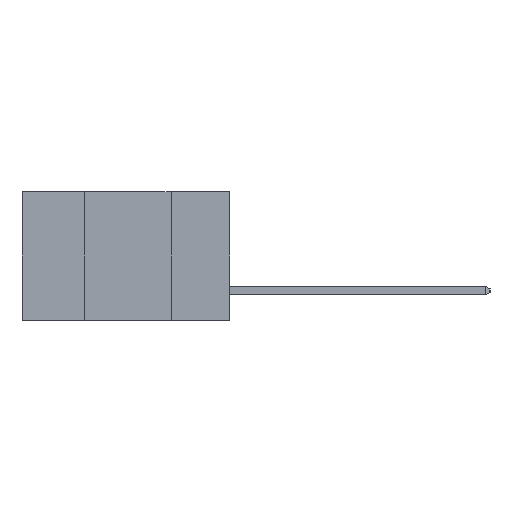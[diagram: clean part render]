
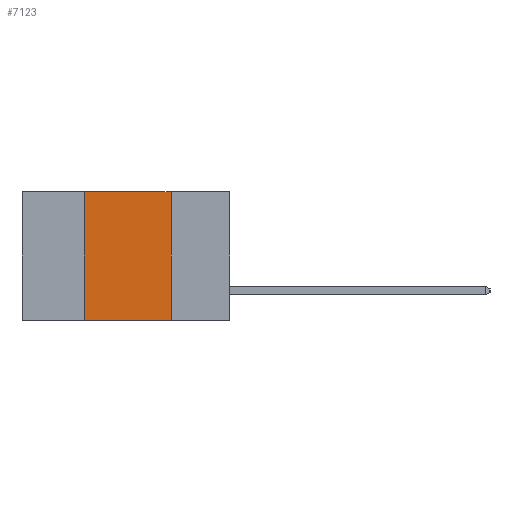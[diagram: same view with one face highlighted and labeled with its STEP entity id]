
A CAD part, left-side view. The second image highlights one B-rep face of the part: STEP entity #7123.
In plain terms, the highlighted planar face has unit normal (-1, 0, 0).
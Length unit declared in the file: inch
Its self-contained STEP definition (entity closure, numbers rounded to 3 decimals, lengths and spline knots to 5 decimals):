
#439 = ORIENTED_EDGE ( 'NONE', *, *, #2695, .F. ) ;
#980 = CARTESIAN_POINT ( 'NONE',  ( 0., 0.6, -0.37 ) ) ;
#1208 = CARTESIAN_POINT ( 'NONE',  ( 0., 0.17, -0.37 ) ) ;
#1499 = CARTESIAN_POINT ( 'NONE',  ( 0., 0.17, 0. ) ) ;
#1862 = DIRECTION ( 'NONE',  ( 1., 0., 0. ) ) ;
#2259 = CARTESIAN_POINT ( 'NONE',  ( 0., 0.42, 0. ) ) ;
#2260 = AXIS2_PLACEMENT_3D ( 'NONE', #10346, #1862, #11417 ) ;
#2314 = CARTESIAN_POINT ( 'NONE',  ( 0., 0.42, 0. ) ) ;
#2387 = DIRECTION ( 'NONE',  ( 0., -1., 0. ) ) ;
#2695 = EDGE_CURVE ( 'NONE', #14999, #3653, #12555, .T. ) ;
#2940 = ORIENTED_EDGE ( 'NONE', *, *, #14162, .F. ) ;
#3653 = VERTEX_POINT ( 'NONE', #1208 ) ;
#3821 = ORIENTED_EDGE ( 'NONE', *, *, #17332, .T. ) ;
#4274 = CARTESIAN_POINT ( 'NONE',  ( 0., 0.17, 0. ) ) ;
#5606 = VECTOR ( 'NONE', #10495, 39.37008 ) ;
#5647 = CARTESIAN_POINT ( 'NONE',  ( 0., 0.42, -0.37 ) ) ;
#7123 = ADVANCED_FACE ( 'NONE', ( #17594 ), #11720, .F. ) ;
#8889 = ORIENTED_EDGE ( 'NONE', *, *, #17670, .F. ) ;
#8890 = VECTOR ( 'NONE', #9823, 39.37008 ) ;
#9500 = CARTESIAN_POINT ( 'NONE',  ( 0., 0.6, 0. ) ) ;
#9823 = DIRECTION ( 'NONE',  ( 0., 0., -1. ) ) ;
#10346 = CARTESIAN_POINT ( 'NONE',  ( 0., 0.6, 0. ) ) ;
#10495 = DIRECTION ( 'NONE',  ( 0., 0., 1. ) ) ;
#10861 = DIRECTION ( 'NONE',  ( 0., -1., 0. ) ) ;
#11157 = VECTOR ( 'NONE', #2387, 39.37008 ) ;
#11417 = DIRECTION ( 'NONE',  ( 0., 0., -1. ) ) ;
#11511 = VERTEX_POINT ( 'NONE', #5647 ) ;
#11592 = LINE ( 'NONE', #980, #11157 ) ;
#11720 = PLANE ( 'NONE',  #2260 ) ;
#12048 = VECTOR ( 'NONE', #10861, 39.37008 ) ;
#12555 = LINE ( 'NONE', #4274, #8890 ) ;
#13047 = EDGE_LOOP ( 'NONE', ( #439, #2940, #8889, #3821 ) ) ;
#14162 = EDGE_CURVE ( 'NONE', #16016, #14999, #16194, .T. ) ;
#14999 = VERTEX_POINT ( 'NONE', #1499 ) ;
#16016 = VERTEX_POINT ( 'NONE', #2314 ) ;
#16194 = LINE ( 'NONE', #9500, #12048 ) ;
#16587 = LINE ( 'NONE', #2259, #5606 ) ;
#17332 = EDGE_CURVE ( 'NONE', #11511, #3653, #11592, .T. ) ;
#17594 = FACE_OUTER_BOUND ( 'NONE', #13047, .T. ) ;
#17670 = EDGE_CURVE ( 'NONE', #11511, #16016, #16587, .T. ) ;
